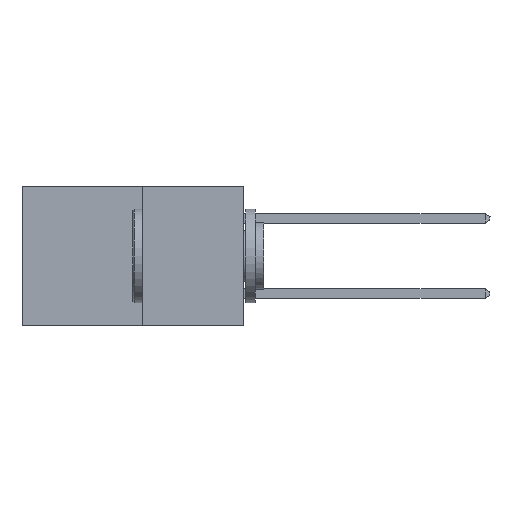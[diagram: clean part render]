
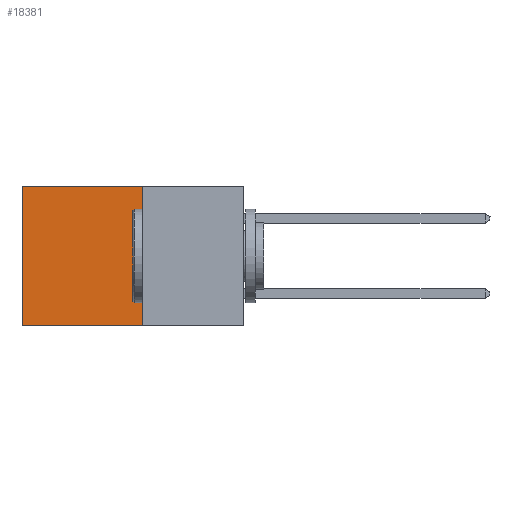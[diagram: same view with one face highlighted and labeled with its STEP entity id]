
A CAD part, left-side view. The second image highlights one B-rep face of the part: STEP entity #18381.
In plain terms, the highlighted planar face has unit normal (-1, 0, 0).
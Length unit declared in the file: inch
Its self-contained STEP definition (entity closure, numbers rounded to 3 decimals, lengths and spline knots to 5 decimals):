
#209 = VERTEX_POINT ( 'NONE', #9112 ) ;
#492 = VECTOR ( 'NONE', #1201, 39.37008 ) ;
#1201 = DIRECTION ( 'NONE',  ( 0., 0., -1. ) ) ;
#1228 = LINE ( 'NONE', #15185, #8555 ) ;
#1705 = CARTESIAN_POINT ( 'NONE',  ( 0.277, 0.59, 0. ) ) ;
#1986 = CARTESIAN_POINT ( 'NONE',  ( 0.277, 0.27, -0.37 ) ) ;
#2148 = ORIENTED_EDGE ( 'NONE', *, *, #15757, .T. ) ;
#3007 = AXIS2_PLACEMENT_3D ( 'NONE', #1986, #7881, #18044 ) ;
#4765 = CARTESIAN_POINT ( 'NONE',  ( 0.277, 0.27, 0. ) ) ;
#5223 = ORIENTED_EDGE ( 'NONE', *, *, #14140, .T. ) ;
#6477 = DIRECTION ( 'NONE',  ( 0., 1., 0. ) ) ;
#6615 = ORIENTED_EDGE ( 'NONE', *, *, #16736, .F. ) ;
#7086 = VECTOR ( 'NONE', #10201, 39.37008 ) ;
#7534 = CARTESIAN_POINT ( 'NONE',  ( 0.277, 0.27, -0.37 ) ) ;
#7881 = DIRECTION ( 'NONE',  ( 1., 0., 0. ) ) ;
#8019 = VERTEX_POINT ( 'NONE', #1705 ) ;
#8555 = VECTOR ( 'NONE', #6477, 39.37008 ) ;
#8726 = CARTESIAN_POINT ( 'NONE',  ( 0.277, 0.27, -0.37 ) ) ;
#8980 = DIRECTION ( 'NONE',  ( 0., 0., -1. ) ) ;
#9112 = CARTESIAN_POINT ( 'NONE',  ( 0.277, 0.59, -0.37 ) ) ;
#9555 = FACE_OUTER_BOUND ( 'NONE', #17226, .T. ) ;
#10201 = DIRECTION ( 'NONE',  ( 0., 1., 0. ) ) ;
#10299 = VECTOR ( 'NONE', #8980, 39.37008 ) ;
#11149 = VERTEX_POINT ( 'NONE', #4765 ) ;
#11176 = ORIENTED_EDGE ( 'NONE', *, *, #17393, .F. ) ;
#13674 = PLANE ( 'NONE',  #3007 ) ;
#14140 = EDGE_CURVE ( 'NONE', #11149, #8019, #1228, .T. ) ;
#15172 = VERTEX_POINT ( 'NONE', #15900 ) ;
#15185 = CARTESIAN_POINT ( 'NONE',  ( 0.277, 0.27, 0. ) ) ;
#15268 = LINE ( 'NONE', #8726, #7086 ) ;
#15757 = EDGE_CURVE ( 'NONE', #8019, #209, #16025, .T. ) ;
#15900 = CARTESIAN_POINT ( 'NONE',  ( 0.277, 0.27, -0.37 ) ) ;
#16025 = LINE ( 'NONE', #18653, #492 ) ;
#16736 = EDGE_CURVE ( 'NONE', #11149, #15172, #18015, .T. ) ;
#17226 = EDGE_LOOP ( 'NONE', ( #2148, #11176, #6615, #5223 ) ) ;
#17393 = EDGE_CURVE ( 'NONE', #15172, #209, #15268, .T. ) ;
#18015 = LINE ( 'NONE', #7534, #10299 ) ;
#18044 = DIRECTION ( 'NONE',  ( 0., 0., -1. ) ) ;
#18381 = ADVANCED_FACE ( 'NONE', ( #9555 ), #13674, .F. ) ;
#18653 = CARTESIAN_POINT ( 'NONE',  ( 0.277, 0.59, -0.37 ) ) ;
